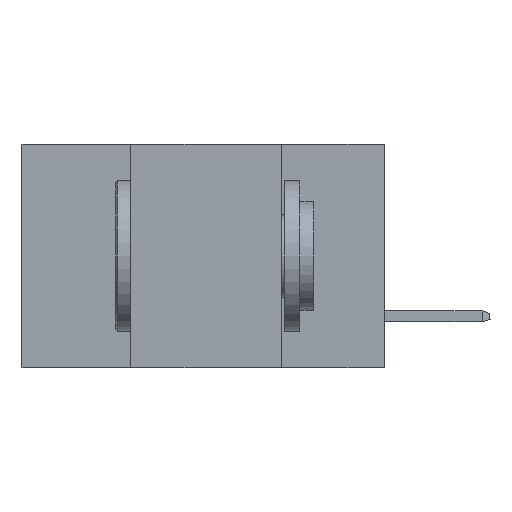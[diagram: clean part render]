
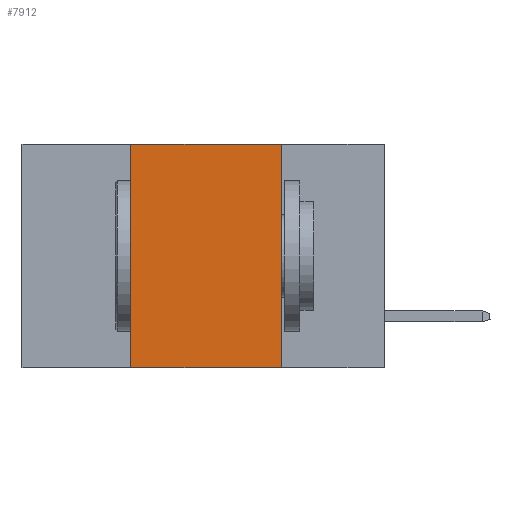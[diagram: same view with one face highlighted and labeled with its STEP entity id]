
A CAD part, left-side view. The second image highlights one B-rep face of the part: STEP entity #7912.
In plain terms, the highlighted planar face has unit normal (-1, 0, 0).
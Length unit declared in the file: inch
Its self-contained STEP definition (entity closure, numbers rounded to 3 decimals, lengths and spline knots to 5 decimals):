
#1559 = EDGE_CURVE ( 'NONE', #21401, #29363, #16416, .T. ) ;
#3025 = DIRECTION ( 'NONE',  ( 1., 0., 0. ) ) ;
#3724 = LINE ( 'NONE', #15966, #23115 ) ;
#5370 = VERTEX_POINT ( 'NONE', #12489 ) ;
#5712 = ORIENTED_EDGE ( 'NONE', *, *, #17155, .F. ) ;
#6081 = ORIENTED_EDGE ( 'NONE', *, *, #1559, .F. ) ;
#6241 = LINE ( 'NONE', #26557, #30653 ) ;
#6616 = FACE_OUTER_BOUND ( 'NONE', #11800, .T. ) ;
#6770 = VECTOR ( 'NONE', #27183, 39.37008 ) ;
#7434 = ORIENTED_EDGE ( 'NONE', *, *, #20485, .T. ) ;
#7912 = ADVANCED_FACE ( 'NONE', ( #6616 ), #25796, .F. ) ;
#8627 = LINE ( 'NONE', #12421, #29894 ) ;
#9845 = CARTESIAN_POINT ( 'NONE',  ( 0., 0.17, 0. ) ) ;
#11203 = DIRECTION ( 'NONE',  ( 0., -1., 0. ) ) ;
#11597 = ORIENTED_EDGE ( 'NONE', *, *, #23109, .F. ) ;
#11800 = EDGE_LOOP ( 'NONE', ( #6081, #5712, #11597, #7434 ) ) ;
#12421 = CARTESIAN_POINT ( 'NONE',  ( 0., 0.6, 0. ) ) ;
#12489 = CARTESIAN_POINT ( 'NONE',  ( 0., 0.42, 0. ) ) ;
#13436 = CARTESIAN_POINT ( 'NONE',  ( 0., 0.6, 0. ) ) ;
#15701 = DIRECTION ( 'NONE',  ( 0., 0., -1. ) ) ;
#15785 = VERTEX_POINT ( 'NONE', #26672 ) ;
#15966 = CARTESIAN_POINT ( 'NONE',  ( 0., 0.6, -0.37 ) ) ;
#16416 = LINE ( 'NONE', #9845, #6770 ) ;
#17155 = EDGE_CURVE ( 'NONE', #5370, #21401, #8627, .T. ) ;
#17931 = DIRECTION ( 'NONE',  ( 0., -1., 0. ) ) ;
#20389 = AXIS2_PLACEMENT_3D ( 'NONE', #13436, #3025, #15701 ) ;
#20485 = EDGE_CURVE ( 'NONE', #15785, #29363, #3724, .T. ) ;
#21351 = CARTESIAN_POINT ( 'NONE',  ( 0., 0.17, -0.37 ) ) ;
#21401 = VERTEX_POINT ( 'NONE', #29658 ) ;
#23109 = EDGE_CURVE ( 'NONE', #15785, #5370, #6241, .T. ) ;
#23115 = VECTOR ( 'NONE', #11203, 39.37008 ) ;
#25796 = PLANE ( 'NONE',  #20389 ) ;
#26557 = CARTESIAN_POINT ( 'NONE',  ( 0., 0.42, 0. ) ) ;
#26672 = CARTESIAN_POINT ( 'NONE',  ( 0., 0.42, -0.37 ) ) ;
#26767 = DIRECTION ( 'NONE',  ( 0., 0., 1. ) ) ;
#27183 = DIRECTION ( 'NONE',  ( 0., 0., -1. ) ) ;
#29363 = VERTEX_POINT ( 'NONE', #21351 ) ;
#29658 = CARTESIAN_POINT ( 'NONE',  ( 0., 0.17, 0. ) ) ;
#29894 = VECTOR ( 'NONE', #17931, 39.37008 ) ;
#30653 = VECTOR ( 'NONE', #26767, 39.37008 ) ;
